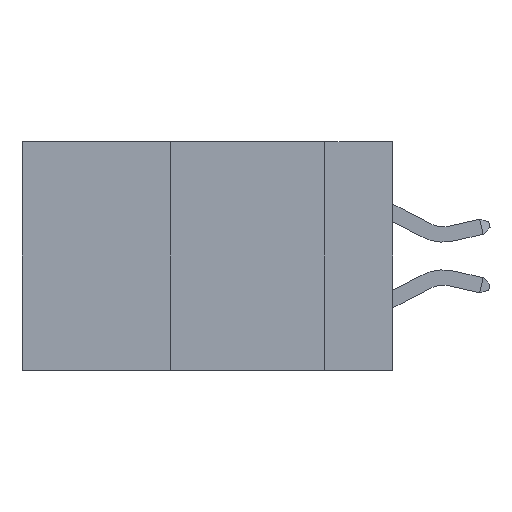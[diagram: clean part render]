
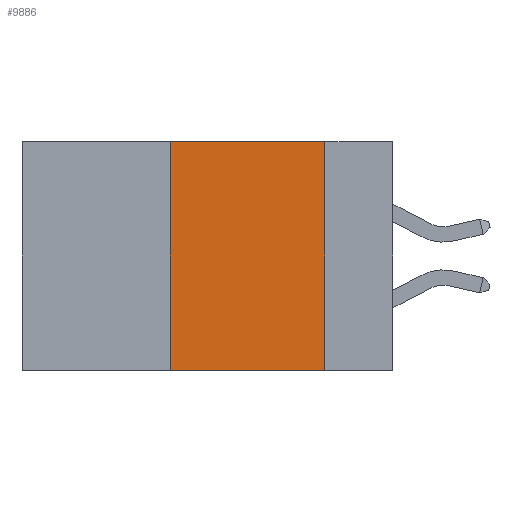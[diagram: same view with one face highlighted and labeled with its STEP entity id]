
A CAD part, left-side view. The second image highlights one B-rep face of the part: STEP entity #9886.
In plain terms, the highlighted planar face has unit normal (-1, 0, 0).
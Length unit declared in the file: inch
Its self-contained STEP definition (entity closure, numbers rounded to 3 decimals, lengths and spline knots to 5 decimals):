
#273 = LINE ( 'NONE', #5793, #3023 ) ;
#425 = CARTESIAN_POINT ( 'NONE',  ( 0., 0.11, 0. ) ) ;
#1206 = DIRECTION ( 'NONE',  ( 1., 0., 0. ) ) ;
#1392 = LINE ( 'NONE', #6067, #8361 ) ;
#1557 = FACE_OUTER_BOUND ( 'NONE', #5270, .T. ) ;
#2133 = PLANE ( 'NONE',  #9281 ) ;
#3023 = VECTOR ( 'NONE', #9330, 39.37008 ) ;
#3027 = ORIENTED_EDGE ( 'NONE', *, *, #8625, .F. ) ;
#3066 = VERTEX_POINT ( 'NONE', #7069 ) ;
#3553 = CARTESIAN_POINT ( 'NONE',  ( 0., 0.11, -0.37 ) ) ;
#3652 = VERTEX_POINT ( 'NONE', #5937 ) ;
#4216 = ORIENTED_EDGE ( 'NONE', *, *, #5852, .T. ) ;
#4844 = ORIENTED_EDGE ( 'NONE', *, *, #9158, .F. ) ;
#5270 = EDGE_LOOP ( 'NONE', ( #4844, #3027, #10350, #4216 ) ) ;
#5587 = VERTEX_POINT ( 'NONE', #3553 ) ;
#5793 = CARTESIAN_POINT ( 'NONE',  ( 0., 0.11, 0. ) ) ;
#5852 = EDGE_CURVE ( 'NONE', #3652, #5587, #6400, .T. ) ;
#5937 = CARTESIAN_POINT ( 'NONE',  ( 0., 0.36, -0.37 ) ) ;
#5974 = DIRECTION ( 'NONE',  ( 0., 0., 1. ) ) ;
#6067 = CARTESIAN_POINT ( 'NONE',  ( 0., 0.36, 0. ) ) ;
#6383 = CARTESIAN_POINT ( 'NONE',  ( 0., 0.6, 0. ) ) ;
#6400 = LINE ( 'NONE', #7277, #10691 ) ;
#6416 = VECTOR ( 'NONE', #10689, 39.37008 ) ;
#6561 = EDGE_CURVE ( 'NONE', #3652, #3066, #1392, .T. ) ;
#6697 = LINE ( 'NONE', #7336, #6416 ) ;
#7069 = CARTESIAN_POINT ( 'NONE',  ( 0., 0.36, 0. ) ) ;
#7277 = CARTESIAN_POINT ( 'NONE',  ( 0., 0.6, -0.37 ) ) ;
#7306 = DIRECTION ( 'NONE',  ( 0., -1., 0. ) ) ;
#7336 = CARTESIAN_POINT ( 'NONE',  ( 0., 0.6, 0. ) ) ;
#7339 = DIRECTION ( 'NONE',  ( 0., 0., -1. ) ) ;
#8361 = VECTOR ( 'NONE', #5974, 39.37008 ) ;
#8625 = EDGE_CURVE ( 'NONE', #3066, #8706, #6697, .T. ) ;
#8706 = VERTEX_POINT ( 'NONE', #425 ) ;
#9158 = EDGE_CURVE ( 'NONE', #8706, #5587, #273, .T. ) ;
#9281 = AXIS2_PLACEMENT_3D ( 'NONE', #6383, #1206, #7339 ) ;
#9330 = DIRECTION ( 'NONE',  ( 0., 0., -1. ) ) ;
#9886 = ADVANCED_FACE ( 'NONE', ( #1557 ), #2133, .F. ) ;
#10350 = ORIENTED_EDGE ( 'NONE', *, *, #6561, .F. ) ;
#10689 = DIRECTION ( 'NONE',  ( 0., -1., 0. ) ) ;
#10691 = VECTOR ( 'NONE', #7306, 39.37008 ) ;
